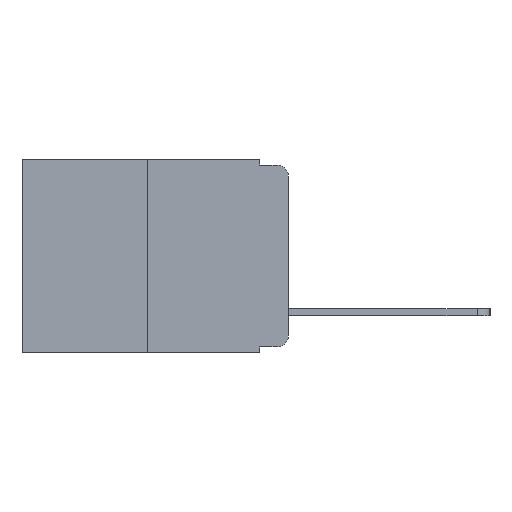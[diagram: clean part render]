
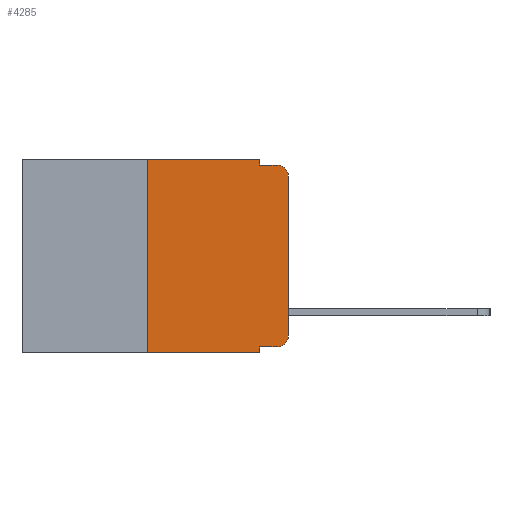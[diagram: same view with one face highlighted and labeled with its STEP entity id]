
A CAD part, left-side view. The second image highlights one B-rep face of the part: STEP entity #4285.
In plain terms, the highlighted planar face has unit normal (-1, 0, 0).
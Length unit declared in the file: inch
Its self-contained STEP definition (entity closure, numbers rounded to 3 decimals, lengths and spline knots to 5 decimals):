
#14 = VECTOR ( 'NONE', #11712, 39.37008 ) ;
#118 = LINE ( 'NONE', #9049, #7445 ) ;
#238 = EDGE_CURVE ( 'NONE', #3127, #6847, #118, .T. ) ;
#556 = EDGE_CURVE ( 'NONE', #9780, #7429, #13966, .T. ) ;
#862 = AXIS2_PLACEMENT_3D ( 'NONE', #16311, #8320, #17588 ) ;
#1232 = VERTEX_POINT ( 'NONE', #10866 ) ;
#1536 = CARTESIAN_POINT ( 'NONE',  ( 0., 0., -0.313 ) ) ;
#1884 = CARTESIAN_POINT ( 'NONE',  ( 0., 0.02, -0.01 ) ) ;
#2076 = CARTESIAN_POINT ( 'NONE',  ( 0., 0.473, 0. ) ) ;
#2148 = ORIENTED_EDGE ( 'NONE', *, *, #8751, .F. ) ;
#2449 = VERTEX_POINT ( 'NONE', #10127 ) ;
#3127 = VERTEX_POINT ( 'NONE', #6471 ) ;
#3634 = DIRECTION ( 'NONE',  ( 0., 0., -1. ) ) ;
#3784 = CARTESIAN_POINT ( 'NONE',  ( 0., 0.02, -0.313 ) ) ;
#4225 = CARTESIAN_POINT ( 'NONE',  ( 0., 0.25, 0. ) ) ;
#4262 = EDGE_CURVE ( 'NONE', #15283, #7429, #12052, .T. ) ;
#4285 = ADVANCED_FACE ( 'NONE', ( #11643 ), #10664, .F. ) ;
#4681 = VECTOR ( 'NONE', #11947, 39.37008 ) ;
#4809 = CARTESIAN_POINT ( 'NONE',  ( 0., 0.051, 0. ) ) ;
#5122 = VECTOR ( 'NONE', #12205, 39.37008 ) ;
#5164 = CARTESIAN_POINT ( 'NONE',  ( 0., 0., 0. ) ) ;
#5176 = ORIENTED_EDGE ( 'NONE', *, *, #7697, .T. ) ;
#5192 = DIRECTION ( 'NONE',  ( 0., 0., -1. ) ) ;
#5281 = DIRECTION ( 'NONE',  ( 0., 0., -1. ) ) ;
#5625 = ORIENTED_EDGE ( 'NONE', *, *, #238, .F. ) ;
#5711 = CARTESIAN_POINT ( 'NONE',  ( 0., 0.051, -0.333 ) ) ;
#6271 = DIRECTION ( 'NONE',  ( 0., 0., -1. ) ) ;
#6311 = VECTOR ( 'NONE', #5192, 39.37008 ) ;
#6463 = AXIS2_PLACEMENT_3D ( 'NONE', #3784, #13457, #5281 ) ;
#6471 = CARTESIAN_POINT ( 'NONE',  ( 0., 0.051, -0.01 ) ) ;
#6522 = ORIENTED_EDGE ( 'NONE', *, *, #9625, .F. ) ;
#6606 = DIRECTION ( 'NONE',  ( 0., 0., 1. ) ) ;
#6653 = VERTEX_POINT ( 'NONE', #10771 ) ;
#6847 = VERTEX_POINT ( 'NONE', #1884 ) ;
#7429 = VERTEX_POINT ( 'NONE', #13084 ) ;
#7445 = VECTOR ( 'NONE', #9187, 39.37008 ) ;
#7572 = VECTOR ( 'NONE', #6606, 39.37008 ) ;
#7631 = AXIS2_PLACEMENT_3D ( 'NONE', #2076, #11999, #3634 ) ;
#7697 = EDGE_CURVE ( 'NONE', #1232, #6847, #11322, .T. ) ;
#7922 = VERTEX_POINT ( 'NONE', #1536 ) ;
#8046 = ORIENTED_EDGE ( 'NONE', *, *, #14692, .T. ) ;
#8184 = CARTESIAN_POINT ( 'NONE',  ( 0., 0.02, -0.333 ) ) ;
#8320 = DIRECTION ( 'NONE',  ( -1., 0., 0. ) ) ;
#8751 = EDGE_CURVE ( 'NONE', #6653, #3127, #16219, .T. ) ;
#9049 = CARTESIAN_POINT ( 'NONE',  ( 0., 0.051, -0.01 ) ) ;
#9187 = DIRECTION ( 'NONE',  ( 0., -1., 0. ) ) ;
#9625 = EDGE_CURVE ( 'NONE', #2449, #6653, #15940, .T. ) ;
#9634 = VERTEX_POINT ( 'NONE', #8184 ) ;
#9780 = VERTEX_POINT ( 'NONE', #5711 ) ;
#10127 = CARTESIAN_POINT ( 'NONE',  ( 0., 0.25, 0. ) ) ;
#10605 = CARTESIAN_POINT ( 'NONE',  ( 0., 0.473, -0.343 ) ) ;
#10616 = ORIENTED_EDGE ( 'NONE', *, *, #13556, .F. ) ;
#10664 = PLANE ( 'NONE',  #7631 ) ;
#10723 = CARTESIAN_POINT ( 'NONE',  ( 0., 0.051, 0. ) ) ;
#10771 = CARTESIAN_POINT ( 'NONE',  ( 0., 0.051, 0. ) ) ;
#10866 = CARTESIAN_POINT ( 'NONE',  ( 0., 0., -0.03 ) ) ;
#10916 = CARTESIAN_POINT ( 'NONE',  ( 0., 0.25, -0.343 ) ) ;
#11322 = CIRCLE ( 'NONE', #862, 0.02 ) ;
#11470 = ORIENTED_EDGE ( 'NONE', *, *, #4262, .T. ) ;
#11643 = FACE_OUTER_BOUND ( 'NONE', #11717, .T. ) ;
#11712 = DIRECTION ( 'NONE',  ( 0., -1., 0. ) ) ;
#11717 = EDGE_LOOP ( 'NONE', ( #15559, #5176, #5625, #2148, #6522, #10616, #11470, #12704, #17817, #8046 ) ) ;
#11947 = DIRECTION ( 'NONE',  ( 0., -1., 0. ) ) ;
#11999 = DIRECTION ( 'NONE',  ( 1., 0., 0. ) ) ;
#12052 = LINE ( 'NONE', #10605, #4681 ) ;
#12099 = VECTOR ( 'NONE', #12534, 39.37008 ) ;
#12205 = DIRECTION ( 'NONE',  ( 0., -1., 0. ) ) ;
#12534 = DIRECTION ( 'NONE',  ( 0., 0., 1. ) ) ;
#12688 = CIRCLE ( 'NONE', #6463, 0.02 ) ;
#12704 = ORIENTED_EDGE ( 'NONE', *, *, #556, .F. ) ;
#13084 = CARTESIAN_POINT ( 'NONE',  ( 0., 0.051, -0.343 ) ) ;
#13457 = DIRECTION ( 'NONE',  ( -1., 0., 0. ) ) ;
#13525 = CARTESIAN_POINT ( 'NONE',  ( 0., 0.473, 0. ) ) ;
#13549 = VECTOR ( 'NONE', #6271, 39.37008 ) ;
#13556 = EDGE_CURVE ( 'NONE', #15283, #2449, #15587, .T. ) ;
#13966 = LINE ( 'NONE', #4809, #13549 ) ;
#14075 = LINE ( 'NONE', #16921, #14 ) ;
#14692 = EDGE_CURVE ( 'NONE', #9634, #7922, #12688, .T. ) ;
#15118 = LINE ( 'NONE', #5164, #7572 ) ;
#15283 = VERTEX_POINT ( 'NONE', #10916 ) ;
#15559 = ORIENTED_EDGE ( 'NONE', *, *, #16347, .T. ) ;
#15587 = LINE ( 'NONE', #4225, #12099 ) ;
#15704 = EDGE_CURVE ( 'NONE', #9780, #9634, #14075, .T. ) ;
#15940 = LINE ( 'NONE', #13525, #5122 ) ;
#16219 = LINE ( 'NONE', #10723, #6311 ) ;
#16311 = CARTESIAN_POINT ( 'NONE',  ( 0., 0.02, -0.03 ) ) ;
#16347 = EDGE_CURVE ( 'NONE', #7922, #1232, #15118, .T. ) ;
#16921 = CARTESIAN_POINT ( 'NONE',  ( 0., 0.051, -0.333 ) ) ;
#17588 = DIRECTION ( 'NONE',  ( 0., 0., -1. ) ) ;
#17817 = ORIENTED_EDGE ( 'NONE', *, *, #15704, .T. ) ;
